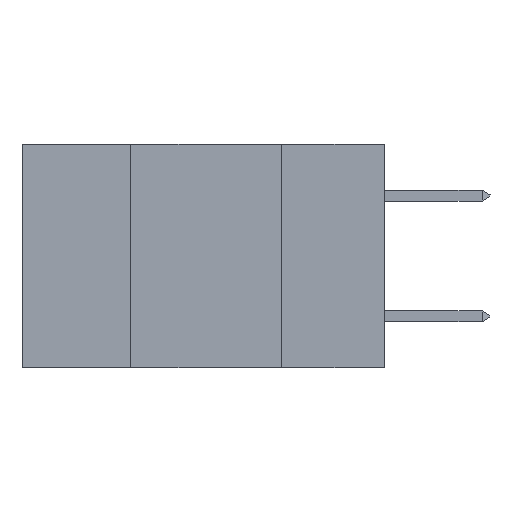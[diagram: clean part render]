
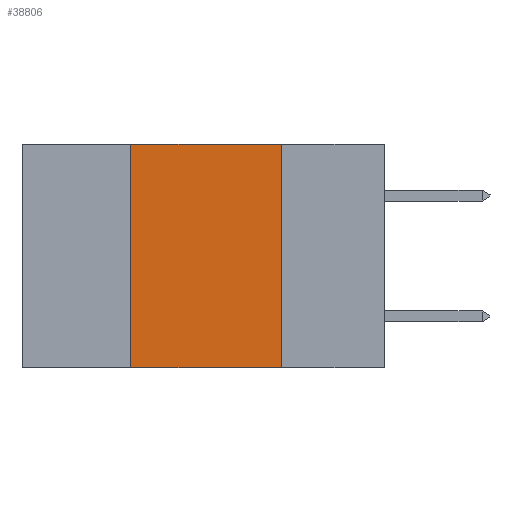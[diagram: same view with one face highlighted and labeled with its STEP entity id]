
A CAD part, left-side view. The second image highlights one B-rep face of the part: STEP entity #38806.
In plain terms, the highlighted planar face has unit normal (-1, 0, 0).
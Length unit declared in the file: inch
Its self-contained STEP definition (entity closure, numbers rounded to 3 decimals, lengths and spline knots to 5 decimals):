
#525 = ORIENTED_EDGE ( 'NONE', *, *, #44585, .F. ) ;
#1059 = LINE ( 'NONE', #5245, #21100 ) ;
#1502 = CARTESIAN_POINT ( 'NONE',  ( 0., 0.42, -0.37 ) ) ;
#1588 = ORIENTED_EDGE ( 'NONE', *, *, #10228, .T. ) ;
#1898 = DIRECTION ( 'NONE',  ( 0., 0., 1. ) ) ;
#4083 = CARTESIAN_POINT ( 'NONE',  ( 0., 0.6, -0.37 ) ) ;
#4990 = VECTOR ( 'NONE', #1898, 39.37008 ) ;
#5203 = CARTESIAN_POINT ( 'NONE',  ( 0., 0.42, 0. ) ) ;
#5245 = CARTESIAN_POINT ( 'NONE',  ( 0., 0.6, 0. ) ) ;
#5323 = VECTOR ( 'NONE', #36011, 39.37008 ) ;
#6183 = ORIENTED_EDGE ( 'NONE', *, *, #21215, .F. ) ;
#8434 = LINE ( 'NONE', #19253, #19840 ) ;
#8936 = VERTEX_POINT ( 'NONE', #40837 ) ;
#10228 = EDGE_CURVE ( 'NONE', #40814, #29969, #42757, .T. ) ;
#10915 = PLANE ( 'NONE',  #40292 ) ;
#13254 = CARTESIAN_POINT ( 'NONE',  ( 0., 0.17, -0.37 ) ) ;
#17907 = CARTESIAN_POINT ( 'NONE',  ( 0., 0.6, 0. ) ) ;
#19253 = CARTESIAN_POINT ( 'NONE',  ( 0., 0.17, 0. ) ) ;
#19840 = VECTOR ( 'NONE', #24016, 39.37008 ) ;
#21100 = VECTOR ( 'NONE', #22541, 39.37008 ) ;
#21215 = EDGE_CURVE ( 'NONE', #8936, #35277, #1059, .T. ) ;
#22541 = DIRECTION ( 'NONE',  ( 0., -1., 0. ) ) ;
#22788 = ORIENTED_EDGE ( 'NONE', *, *, #31151, .F. ) ;
#24016 = DIRECTION ( 'NONE',  ( 0., 0., -1. ) ) ;
#25033 = DIRECTION ( 'NONE',  ( 0., 0., -1. ) ) ;
#27235 = FACE_OUTER_BOUND ( 'NONE', #40863, .T. ) ;
#28396 = DIRECTION ( 'NONE',  ( 1., 0., 0. ) ) ;
#29969 = VERTEX_POINT ( 'NONE', #13254 ) ;
#31151 = EDGE_CURVE ( 'NONE', #35277, #29969, #8434, .T. ) ;
#35277 = VERTEX_POINT ( 'NONE', #41733 ) ;
#36011 = DIRECTION ( 'NONE',  ( 0., -1., 0. ) ) ;
#37482 = LINE ( 'NONE', #5203, #4990 ) ;
#38806 = ADVANCED_FACE ( 'NONE', ( #27235 ), #10915, .F. ) ;
#40292 = AXIS2_PLACEMENT_3D ( 'NONE', #17907, #28396, #25033 ) ;
#40814 = VERTEX_POINT ( 'NONE', #1502 ) ;
#40837 = CARTESIAN_POINT ( 'NONE',  ( 0., 0.42, 0. ) ) ;
#40863 = EDGE_LOOP ( 'NONE', ( #22788, #6183, #525, #1588 ) ) ;
#41733 = CARTESIAN_POINT ( 'NONE',  ( 0., 0.17, 0. ) ) ;
#42757 = LINE ( 'NONE', #4083, #5323 ) ;
#44585 = EDGE_CURVE ( 'NONE', #40814, #8936, #37482, .T. ) ;
